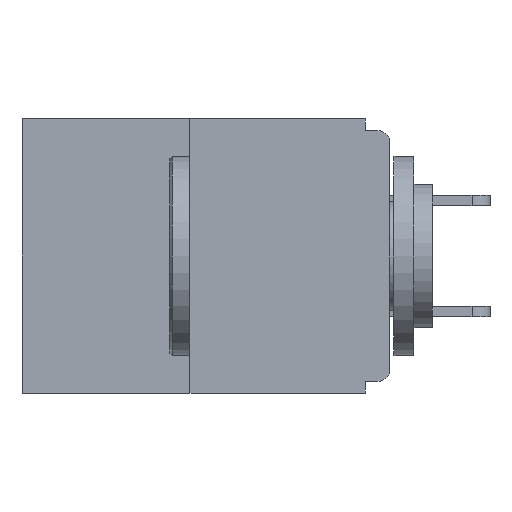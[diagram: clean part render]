
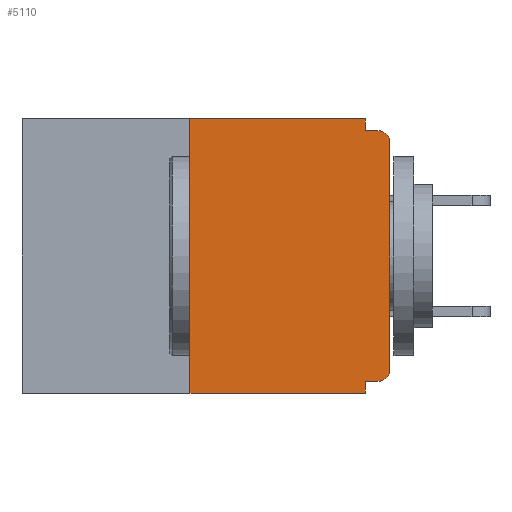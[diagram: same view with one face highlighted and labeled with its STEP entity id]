
A CAD part, left-side view. The second image highlights one B-rep face of the part: STEP entity #5110.
In plain terms, the highlighted planar face has unit normal (-1, 0, 0).
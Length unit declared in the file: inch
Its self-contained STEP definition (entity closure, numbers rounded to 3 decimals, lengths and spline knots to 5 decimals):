
#244 = CARTESIAN_POINT ( 'NONE',  ( 0., 0., -0.313 ) ) ;
#276 = VERTEX_POINT ( 'NONE', #11640 ) ;
#521 = DIRECTION ( 'NONE',  ( 0., 0., -1. ) ) ;
#725 = VERTEX_POINT ( 'NONE', #11832 ) ;
#1084 = VECTOR ( 'NONE', #14046, 39.37008 ) ;
#1446 = DIRECTION ( 'NONE',  ( 0., 0., -1. ) ) ;
#1987 = LINE ( 'NONE', #14257, #13675 ) ;
#2175 = ORIENTED_EDGE ( 'NONE', *, *, #16574, .F. ) ;
#2298 = DIRECTION ( 'NONE',  ( -1., 0., 0. ) ) ;
#2330 = CARTESIAN_POINT ( 'NONE',  ( 0., 0.015, -0.015 ) ) ;
#2442 = CARTESIAN_POINT ( 'NONE',  ( 0., 0.25, 0. ) ) ;
#2460 = ORIENTED_EDGE ( 'NONE', *, *, #21062, .F. ) ;
#2760 = DIRECTION ( 'NONE',  ( 0., 0., -1. ) ) ;
#3141 = DIRECTION ( 'NONE',  ( 0., 1., 0. ) ) ;
#3918 = DIRECTION ( 'NONE',  ( 0., 0., 1. ) ) ;
#4052 = EDGE_CURVE ( 'NONE', #15857, #7719, #20657, .T. ) ;
#4240 = VECTOR ( 'NONE', #4313, 39.37008 ) ;
#4286 = FACE_OUTER_BOUND ( 'NONE', #4731, .T. ) ;
#4313 = DIRECTION ( 'NONE',  ( 0., 0., -1. ) ) ;
#4358 = EDGE_CURVE ( 'NONE', #18346, #17502, #8970, .T. ) ;
#4460 = CARTESIAN_POINT ( 'NONE',  ( 0., 0.46, 0. ) ) ;
#4511 = VERTEX_POINT ( 'NONE', #2442 ) ;
#4602 = DIRECTION ( 'NONE',  ( 0., -1., 0. ) ) ;
#4731 = EDGE_LOOP ( 'NONE', ( #15086, #10908, #7066, #2460, #10790, #4802, #17379, #17629, #14933, #2175 ) ) ;
#4802 = ORIENTED_EDGE ( 'NONE', *, *, #4358, .T. ) ;
#4820 = CARTESIAN_POINT ( 'NONE',  ( 0., 0.031, -0.343 ) ) ;
#5024 = LINE ( 'NONE', #17607, #4240 ) ;
#5110 = ADVANCED_FACE ( 'NONE', ( #4286 ), #15614, .F. ) ;
#5524 = VECTOR ( 'NONE', #1446, 39.37008 ) ;
#5734 = DIRECTION ( 'NONE',  ( 0., -1., 0. ) ) ;
#5742 = CARTESIAN_POINT ( 'NONE',  ( 0., 0.015, -0.313 ) ) ;
#6021 = EDGE_CURVE ( 'NONE', #18346, #18816, #6561, .T. ) ;
#6078 = AXIS2_PLACEMENT_3D ( 'NONE', #5742, #2298, #521 ) ;
#6561 = LINE ( 'NONE', #6564, #16388 ) ;
#6564 = CARTESIAN_POINT ( 'NONE',  ( 0., 0., -0.328 ) ) ;
#7066 = ORIENTED_EDGE ( 'NONE', *, *, #11101, .T. ) ;
#7289 = CARTESIAN_POINT ( 'NONE',  ( 0., 0.46, 0. ) ) ;
#7362 = DIRECTION ( 'NONE',  ( 1., 0., 0. ) ) ;
#7629 = VECTOR ( 'NONE', #4602, 39.37008 ) ;
#7719 = VERTEX_POINT ( 'NONE', #2330 ) ;
#8397 = LINE ( 'NONE', #14605, #13866 ) ;
#8970 = CIRCLE ( 'NONE', #6078, 0.015 ) ;
#9030 = VECTOR ( 'NONE', #3918, 39.37008 ) ;
#9093 = EDGE_CURVE ( 'NONE', #276, #4511, #13444, .T. ) ;
#9781 = VERTEX_POINT ( 'NONE', #19821 ) ;
#10790 = ORIENTED_EDGE ( 'NONE', *, *, #6021, .F. ) ;
#10908 = ORIENTED_EDGE ( 'NONE', *, *, #9093, .F. ) ;
#11101 = EDGE_CURVE ( 'NONE', #276, #13331, #8397, .T. ) ;
#11117 = DIRECTION ( 'NONE',  ( -1., 0., 0. ) ) ;
#11467 = DIRECTION ( 'NONE',  ( 0., -1., 0. ) ) ;
#11640 = CARTESIAN_POINT ( 'NONE',  ( 0., 0.25, -0.343 ) ) ;
#11832 = CARTESIAN_POINT ( 'NONE',  ( 0., 0.031, -0.015 ) ) ;
#12042 = LINE ( 'NONE', #4460, #7629 ) ;
#12268 = EDGE_CURVE ( 'NONE', #17502, #15857, #14842, .T. ) ;
#13331 = VERTEX_POINT ( 'NONE', #21384 ) ;
#13444 = LINE ( 'NONE', #13929, #9030 ) ;
#13675 = VECTOR ( 'NONE', #5734, 39.37008 ) ;
#13866 = VECTOR ( 'NONE', #11467, 39.37008 ) ;
#13929 = CARTESIAN_POINT ( 'NONE',  ( 0., 0.25, 0. ) ) ;
#14046 = DIRECTION ( 'NONE',  ( 0., 0., 1. ) ) ;
#14257 = CARTESIAN_POINT ( 'NONE',  ( 0., 0., -0.015 ) ) ;
#14459 = EDGE_CURVE ( 'NONE', #4511, #9781, #12042, .T. ) ;
#14605 = CARTESIAN_POINT ( 'NONE',  ( 0., 0.46, -0.343 ) ) ;
#14842 = LINE ( 'NONE', #20631, #1084 ) ;
#14933 = ORIENTED_EDGE ( 'NONE', *, *, #19183, .F. ) ;
#15086 = ORIENTED_EDGE ( 'NONE', *, *, #14459, .F. ) ;
#15463 = CARTESIAN_POINT ( 'NONE',  ( 0., 0.031, -0.328 ) ) ;
#15614 = PLANE ( 'NONE',  #19238 ) ;
#15857 = VERTEX_POINT ( 'NONE', #17935 ) ;
#16388 = VECTOR ( 'NONE', #3141, 39.37008 ) ;
#16574 = EDGE_CURVE ( 'NONE', #9781, #725, #5024, .T. ) ;
#17379 = ORIENTED_EDGE ( 'NONE', *, *, #12268, .T. ) ;
#17502 = VERTEX_POINT ( 'NONE', #244 ) ;
#17607 = CARTESIAN_POINT ( 'NONE',  ( 0., 0.031, 0. ) ) ;
#17629 = ORIENTED_EDGE ( 'NONE', *, *, #4052, .T. ) ;
#17935 = CARTESIAN_POINT ( 'NONE',  ( 0., 0., -0.03 ) ) ;
#18346 = VERTEX_POINT ( 'NONE', #18989 ) ;
#18816 = VERTEX_POINT ( 'NONE', #15463 ) ;
#18989 = CARTESIAN_POINT ( 'NONE',  ( 0., 0.015, -0.328 ) ) ;
#19183 = EDGE_CURVE ( 'NONE', #725, #7719, #1987, .T. ) ;
#19238 = AXIS2_PLACEMENT_3D ( 'NONE', #7289, #7362, #2760 ) ;
#19386 = CARTESIAN_POINT ( 'NONE',  ( 0., 0.015, -0.03 ) ) ;
#19821 = CARTESIAN_POINT ( 'NONE',  ( 0., 0.031, 0. ) ) ;
#19991 = LINE ( 'NONE', #4820, #5524 ) ;
#20631 = CARTESIAN_POINT ( 'NONE',  ( 0., 0., 0. ) ) ;
#20657 = CIRCLE ( 'NONE', #21192, 0.015 ) ;
#21062 = EDGE_CURVE ( 'NONE', #18816, #13331, #19991, .T. ) ;
#21067 = DIRECTION ( 'NONE',  ( 0., 0., -1. ) ) ;
#21192 = AXIS2_PLACEMENT_3D ( 'NONE', #19386, #11117, #21067 ) ;
#21384 = CARTESIAN_POINT ( 'NONE',  ( 0., 0.031, -0.343 ) ) ;
